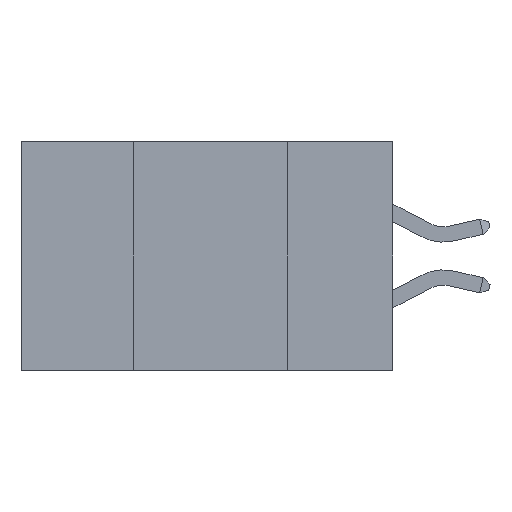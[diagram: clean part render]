
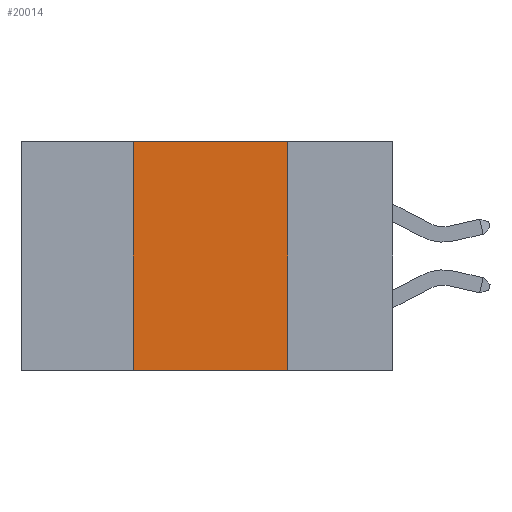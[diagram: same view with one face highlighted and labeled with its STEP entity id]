
A CAD part, left-side view. The second image highlights one B-rep face of the part: STEP entity #20014.
In plain terms, the highlighted planar face has unit normal (-1, 0, 0).
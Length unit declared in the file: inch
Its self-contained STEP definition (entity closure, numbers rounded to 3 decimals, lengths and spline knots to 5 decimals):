
#746 = ORIENTED_EDGE ( 'NONE', *, *, #19169, .T. ) ;
#784 = LINE ( 'NONE', #6863, #2820 ) ;
#1920 = CARTESIAN_POINT ( 'NONE',  ( 0., 0.6, -0.37 ) ) ;
#2598 = DIRECTION ( 'NONE',  ( 0., 0., -1. ) ) ;
#2820 = VECTOR ( 'NONE', #19999, 39.37008 ) ;
#4941 = LINE ( 'NONE', #6378, #10165 ) ;
#5592 = VERTEX_POINT ( 'NONE', #14321 ) ;
#6134 = CARTESIAN_POINT ( 'NONE',  ( 0., 0.6, 0. ) ) ;
#6282 = VECTOR ( 'NONE', #22741, 39.37008 ) ;
#6378 = CARTESIAN_POINT ( 'NONE',  ( 0., 0.42, 0. ) ) ;
#6863 = CARTESIAN_POINT ( 'NONE',  ( 0., 0.6, 0. ) ) ;
#7046 = VECTOR ( 'NONE', #20880, 39.37008 ) ;
#7459 = ORIENTED_EDGE ( 'NONE', *, *, #15961, .F. ) ;
#7529 = VERTEX_POINT ( 'NONE', #22491 ) ;
#8119 = PLANE ( 'NONE',  #16191 ) ;
#8980 = CARTESIAN_POINT ( 'NONE',  ( 0., 0.42, -0.37 ) ) ;
#9532 = VERTEX_POINT ( 'NONE', #16654 ) ;
#10165 = VECTOR ( 'NONE', #23234, 39.37008 ) ;
#11809 = EDGE_CURVE ( 'NONE', #9532, #5592, #18394, .T. ) ;
#12019 = LINE ( 'NONE', #1920, #7046 ) ;
#14321 = CARTESIAN_POINT ( 'NONE',  ( 0., 0.17, -0.37 ) ) ;
#15414 = EDGE_CURVE ( 'NONE', #16568, #7529, #4941, .T. ) ;
#15961 = EDGE_CURVE ( 'NONE', #7529, #9532, #784, .T. ) ;
#16191 = AXIS2_PLACEMENT_3D ( 'NONE', #6134, #21081, #2598 ) ;
#16568 = VERTEX_POINT ( 'NONE', #8980 ) ;
#16654 = CARTESIAN_POINT ( 'NONE',  ( 0., 0.17, 0. ) ) ;
#17745 = ORIENTED_EDGE ( 'NONE', *, *, #15414, .F. ) ;
#18324 = ORIENTED_EDGE ( 'NONE', *, *, #11809, .F. ) ;
#18394 = LINE ( 'NONE', #20846, #6282 ) ;
#19169 = EDGE_CURVE ( 'NONE', #16568, #5592, #12019, .T. ) ;
#19362 = FACE_OUTER_BOUND ( 'NONE', #24210, .T. ) ;
#19999 = DIRECTION ( 'NONE',  ( 0., -1., 0. ) ) ;
#20014 = ADVANCED_FACE ( 'NONE', ( #19362 ), #8119, .F. ) ;
#20846 = CARTESIAN_POINT ( 'NONE',  ( 0., 0.17, 0. ) ) ;
#20880 = DIRECTION ( 'NONE',  ( 0., -1., 0. ) ) ;
#21081 = DIRECTION ( 'NONE',  ( 1., 0., 0. ) ) ;
#22491 = CARTESIAN_POINT ( 'NONE',  ( 0., 0.42, 0. ) ) ;
#22741 = DIRECTION ( 'NONE',  ( 0., 0., -1. ) ) ;
#23234 = DIRECTION ( 'NONE',  ( 0., 0., 1. ) ) ;
#24210 = EDGE_LOOP ( 'NONE', ( #18324, #7459, #17745, #746 ) ) ;
